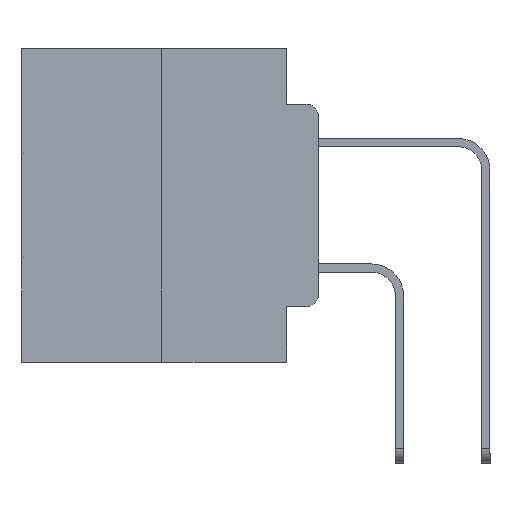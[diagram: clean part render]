
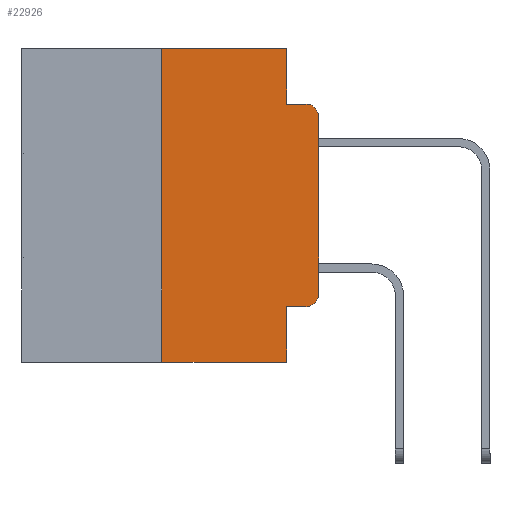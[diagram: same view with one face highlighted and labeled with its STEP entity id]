
A CAD part, left-side view. The second image highlights one B-rep face of the part: STEP entity #22926.
In plain terms, the highlighted planar face has unit normal (-1, 0, 0).
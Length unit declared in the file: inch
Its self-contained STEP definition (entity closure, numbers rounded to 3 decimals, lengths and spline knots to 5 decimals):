
#63 = EDGE_CURVE ( 'NONE', #22785, #20558, #6986, .T. ) ;
#284 = ORIENTED_EDGE ( 'NONE', *, *, #28102, .T. ) ;
#305 = VECTOR ( 'NONE', #7681, 39.37008 ) ;
#653 = EDGE_CURVE ( 'NONE', #27677, #4280, #18037, .T. ) ;
#731 = VECTOR ( 'NONE', #1110, 39.37008 ) ;
#1030 = LINE ( 'NONE', #5568, #305 ) ;
#1110 = DIRECTION ( 'NONE',  ( 0., -1., 0. ) ) ;
#1251 = LINE ( 'NONE', #14781, #18256 ) ;
#1558 = VECTOR ( 'NONE', #19922, 39.37008 ) ;
#1943 = CARTESIAN_POINT ( 'NONE',  ( 0., 0.051, -0.0885 ) ) ;
#2103 = DIRECTION ( 'NONE',  ( 0., 0., -1. ) ) ;
#2581 = DIRECTION ( 'NONE',  ( 0., 0., -1. ) ) ;
#2598 = EDGE_CURVE ( 'NONE', #27457, #17163, #1251, .T. ) ;
#2814 = VECTOR ( 'NONE', #2103, 39.37008 ) ;
#2927 = PLANE ( 'NONE',  #6840 ) ;
#3462 = CARTESIAN_POINT ( 'NONE',  ( 0., 0.02, -0.3915 ) ) ;
#3691 = VERTEX_POINT ( 'NONE', #13358 ) ;
#4280 = VERTEX_POINT ( 'NONE', #26221 ) ;
#4356 = CARTESIAN_POINT ( 'NONE',  ( 0., 0.25, -0.5 ) ) ;
#4617 = CARTESIAN_POINT ( 'NONE',  ( 0., 0.02, -0.1085 ) ) ;
#4855 = ORIENTED_EDGE ( 'NONE', *, *, #6563, .T. ) ;
#5243 = CARTESIAN_POINT ( 'NONE',  ( 0., 0.051, -0.4115 ) ) ;
#5568 = CARTESIAN_POINT ( 'NONE',  ( 0., 0.051, -0.0885 ) ) ;
#6563 = EDGE_CURVE ( 'NONE', #27457, #4280, #13838, .T. ) ;
#6683 = LINE ( 'NONE', #16582, #731 ) ;
#6740 = CARTESIAN_POINT ( 'NONE',  ( 0., 0., 0. ) ) ;
#6840 = AXIS2_PLACEMENT_3D ( 'NONE', #7414, #22740, #9630 ) ;
#6846 = DIRECTION ( 'NONE',  ( 0., 0., -1. ) ) ;
#6986 = CIRCLE ( 'NONE', #7743, 0.02 ) ;
#7414 = CARTESIAN_POINT ( 'NONE',  ( 0., 0.473, 0. ) ) ;
#7681 = DIRECTION ( 'NONE',  ( 0., -1., 0. ) ) ;
#7743 = AXIS2_PLACEMENT_3D ( 'NONE', #3462, #18015, #2581 ) ;
#8170 = CARTESIAN_POINT ( 'NONE',  ( 0., 0., -0.1085 ) ) ;
#8648 = VECTOR ( 'NONE', #27715, 39.37008 ) ;
#8666 = ORIENTED_EDGE ( 'NONE', *, *, #2598, .F. ) ;
#8669 = CARTESIAN_POINT ( 'NONE',  ( 0., 0.051, 0. ) ) ;
#8808 = VERTEX_POINT ( 'NONE', #1943 ) ;
#9271 = ORIENTED_EDGE ( 'NONE', *, *, #14934, .T. ) ;
#9381 = VERTEX_POINT ( 'NONE', #8170 ) ;
#9630 = DIRECTION ( 'NONE',  ( 0., 0., -1. ) ) ;
#10055 = VECTOR ( 'NONE', #14659, 39.37008 ) ;
#10690 = CIRCLE ( 'NONE', #25426, 0.02 ) ;
#11153 = EDGE_CURVE ( 'NONE', #17163, #22781, #6683, .T. ) ;
#11201 = CARTESIAN_POINT ( 'NONE',  ( 0., 0.25, 0. ) ) ;
#12141 = ORIENTED_EDGE ( 'NONE', *, *, #26365, .F. ) ;
#13358 = CARTESIAN_POINT ( 'NONE',  ( 0., 0.02, -0.0885 ) ) ;
#13378 = LINE ( 'NONE', #6740, #1558 ) ;
#13641 = DIRECTION ( 'NONE',  ( 0., -1., 0. ) ) ;
#13838 = LINE ( 'NONE', #26599, #20330 ) ;
#14391 = DIRECTION ( 'NONE',  ( 0., 0., 1. ) ) ;
#14659 = DIRECTION ( 'NONE',  ( 0., 0., -1. ) ) ;
#14781 = CARTESIAN_POINT ( 'NONE',  ( 0., 0.25, 0. ) ) ;
#14934 = EDGE_CURVE ( 'NONE', #27677, #22785, #15252, .T. ) ;
#15252 = LINE ( 'NONE', #25564, #8648 ) ;
#16207 = ORIENTED_EDGE ( 'NONE', *, *, #63, .T. ) ;
#16582 = CARTESIAN_POINT ( 'NONE',  ( 0., 0.473, 0. ) ) ;
#17163 = VERTEX_POINT ( 'NONE', #11201 ) ;
#17361 = ORIENTED_EDGE ( 'NONE', *, *, #27127, .F. ) ;
#17662 = EDGE_CURVE ( 'NONE', #20558, #9381, #13378, .T. ) ;
#17964 = CARTESIAN_POINT ( 'NONE',  ( 0., 0.02, -0.4115 ) ) ;
#18015 = DIRECTION ( 'NONE',  ( -1., 0., 0. ) ) ;
#18037 = LINE ( 'NONE', #8669, #10055 ) ;
#18256 = VECTOR ( 'NONE', #14391, 39.37008 ) ;
#19789 = CARTESIAN_POINT ( 'NONE',  ( 0., 0.051, 0. ) ) ;
#19834 = CARTESIAN_POINT ( 'NONE',  ( 0., 0.051, 0. ) ) ;
#19918 = FACE_OUTER_BOUND ( 'NONE', #26849, .T. ) ;
#19922 = DIRECTION ( 'NONE',  ( 0., 0., 1. ) ) ;
#20025 = DIRECTION ( 'NONE',  ( -1., 0., 0. ) ) ;
#20330 = VECTOR ( 'NONE', #13641, 39.37008 ) ;
#20558 = VERTEX_POINT ( 'NONE', #23913 ) ;
#22740 = DIRECTION ( 'NONE',  ( 1., 0., 0. ) ) ;
#22781 = VERTEX_POINT ( 'NONE', #19834 ) ;
#22785 = VERTEX_POINT ( 'NONE', #17964 ) ;
#22926 = ADVANCED_FACE ( 'NONE', ( #19918 ), #2927, .F. ) ;
#23913 = CARTESIAN_POINT ( 'NONE',  ( 0., 0., -0.3915 ) ) ;
#25403 = ORIENTED_EDGE ( 'NONE', *, *, #17662, .T. ) ;
#25426 = AXIS2_PLACEMENT_3D ( 'NONE', #4617, #20025, #6846 ) ;
#25564 = CARTESIAN_POINT ( 'NONE',  ( 0., 0.051, -0.4115 ) ) ;
#25984 = ORIENTED_EDGE ( 'NONE', *, *, #653, .F. ) ;
#26075 = ORIENTED_EDGE ( 'NONE', *, *, #11153, .F. ) ;
#26146 = LINE ( 'NONE', #19789, #2814 ) ;
#26221 = CARTESIAN_POINT ( 'NONE',  ( 0., 0.051, -0.5 ) ) ;
#26365 = EDGE_CURVE ( 'NONE', #22781, #8808, #26146, .T. ) ;
#26599 = CARTESIAN_POINT ( 'NONE',  ( 0., 0.473, -0.5 ) ) ;
#26849 = EDGE_LOOP ( 'NONE', ( #25403, #284, #17361, #12141, #26075, #8666, #4855, #25984, #9271, #16207 ) ) ;
#27127 = EDGE_CURVE ( 'NONE', #8808, #3691, #1030, .T. ) ;
#27457 = VERTEX_POINT ( 'NONE', #4356 ) ;
#27677 = VERTEX_POINT ( 'NONE', #5243 ) ;
#27715 = DIRECTION ( 'NONE',  ( 0., -1., 0. ) ) ;
#28102 = EDGE_CURVE ( 'NONE', #9381, #3691, #10690, .T. ) ;
